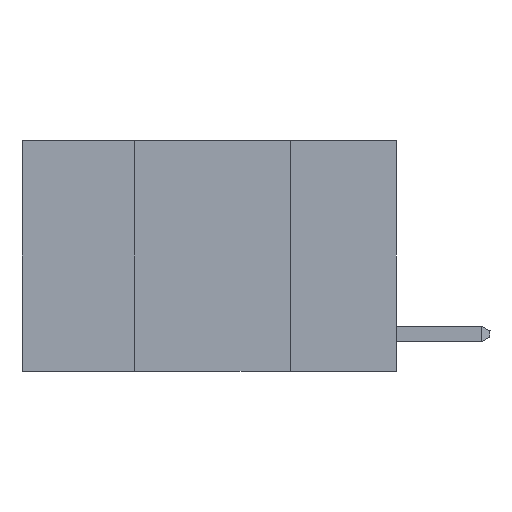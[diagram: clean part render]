
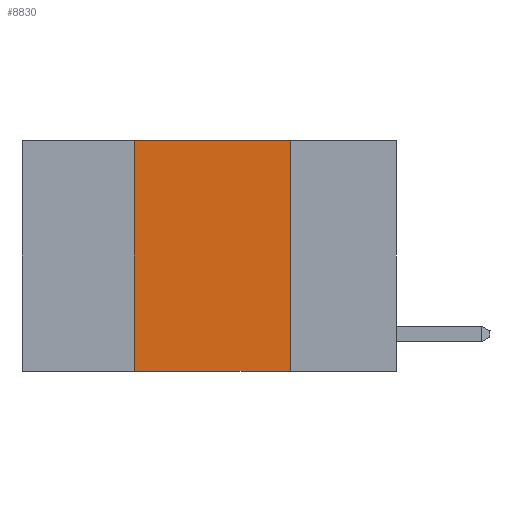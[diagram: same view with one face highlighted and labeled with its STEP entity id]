
A CAD part, left-side view. The second image highlights one B-rep face of the part: STEP entity #8830.
In plain terms, the highlighted planar face has unit normal (-1, 0, 0).
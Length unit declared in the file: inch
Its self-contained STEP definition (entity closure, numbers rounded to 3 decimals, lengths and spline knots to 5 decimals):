
#1146 = AXIS2_PLACEMENT_3D ( 'NONE', #10531, #14569, #13288 ) ;
#2048 = DIRECTION ( 'NONE',  ( 0., 0., 1. ) ) ;
#3284 = VERTEX_POINT ( 'NONE', #5885 ) ;
#3766 = ORIENTED_EDGE ( 'NONE', *, *, #11875, .T. ) ;
#3943 = FACE_OUTER_BOUND ( 'NONE', #10321, .T. ) ;
#4135 = CARTESIAN_POINT ( 'NONE',  ( 0., 0.42, -0.37 ) ) ;
#4163 = EDGE_CURVE ( 'NONE', #3284, #5092, #12333, .T. ) ;
#4550 = LINE ( 'NONE', #7203, #5291 ) ;
#4698 = CARTESIAN_POINT ( 'NONE',  ( 0., 0.17, 0. ) ) ;
#5092 = VERTEX_POINT ( 'NONE', #8850 ) ;
#5291 = VECTOR ( 'NONE', #12432, 39.37008 ) ;
#5885 = CARTESIAN_POINT ( 'NONE',  ( 0., 0.17, 0. ) ) ;
#6197 = VECTOR ( 'NONE', #14213, 39.37008 ) ;
#6497 = CARTESIAN_POINT ( 'NONE',  ( 0., 0.6, 0. ) ) ;
#6503 = ORIENTED_EDGE ( 'NONE', *, *, #12250, .F. ) ;
#6603 = PLANE ( 'NONE',  #1146 ) ;
#7074 = LINE ( 'NONE', #7330, #13248 ) ;
#7203 = CARTESIAN_POINT ( 'NONE',  ( 0., 0.6, -0.37 ) ) ;
#7330 = CARTESIAN_POINT ( 'NONE',  ( 0., 0.42, 0. ) ) ;
#8633 = DIRECTION ( 'NONE',  ( 0., 0., -1. ) ) ;
#8830 = ADVANCED_FACE ( 'NONE', ( #3943 ), #6603, .F. ) ;
#8850 = CARTESIAN_POINT ( 'NONE',  ( 0., 0.17, -0.37 ) ) ;
#10321 = EDGE_LOOP ( 'NONE', ( #13297, #14214, #6503, #3766 ) ) ;
#10531 = CARTESIAN_POINT ( 'NONE',  ( 0., 0.6, 0. ) ) ;
#11875 = EDGE_CURVE ( 'NONE', #14335, #5092, #4550, .T. ) ;
#12250 = EDGE_CURVE ( 'NONE', #14335, #12513, #7074, .T. ) ;
#12333 = LINE ( 'NONE', #4698, #13846 ) ;
#12432 = DIRECTION ( 'NONE',  ( 0., -1., 0. ) ) ;
#12513 = VERTEX_POINT ( 'NONE', #14439 ) ;
#13248 = VECTOR ( 'NONE', #2048, 39.37008 ) ;
#13288 = DIRECTION ( 'NONE',  ( 0., 0., -1. ) ) ;
#13297 = ORIENTED_EDGE ( 'NONE', *, *, #4163, .F. ) ;
#13846 = VECTOR ( 'NONE', #8633, 39.37008 ) ;
#14213 = DIRECTION ( 'NONE',  ( 0., -1., 0. ) ) ;
#14214 = ORIENTED_EDGE ( 'NONE', *, *, #16758, .F. ) ;
#14335 = VERTEX_POINT ( 'NONE', #4135 ) ;
#14439 = CARTESIAN_POINT ( 'NONE',  ( 0., 0.42, 0. ) ) ;
#14569 = DIRECTION ( 'NONE',  ( 1., 0., 0. ) ) ;
#16758 = EDGE_CURVE ( 'NONE', #12513, #3284, #16886, .T. ) ;
#16886 = LINE ( 'NONE', #6497, #6197 ) ;
